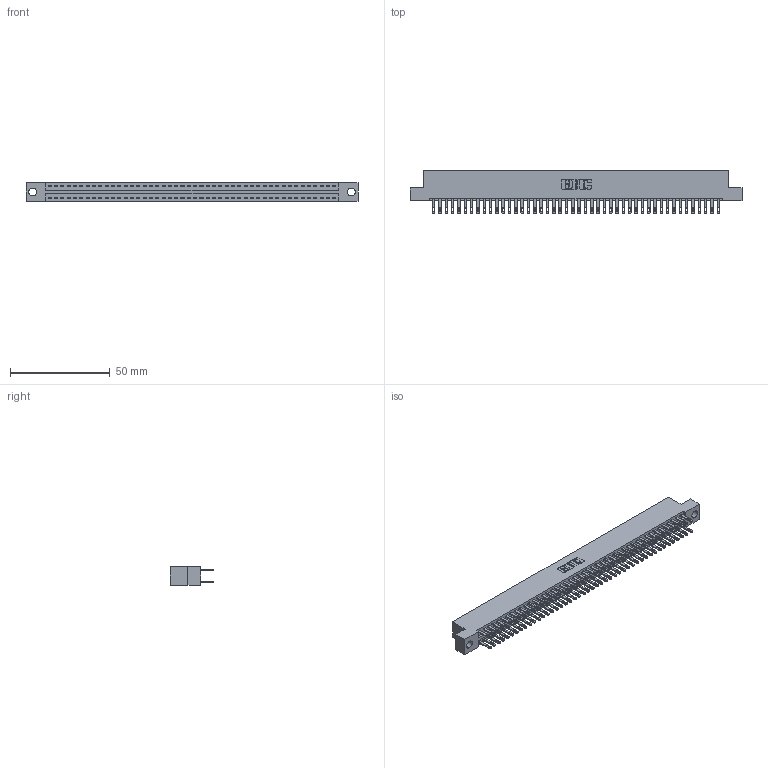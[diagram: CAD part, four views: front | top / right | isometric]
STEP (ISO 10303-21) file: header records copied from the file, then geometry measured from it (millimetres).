
FILE_DESCRIPTION (( 'STEP AP203' ), '1' );
FILE_NAME ('346-092-500-204.STEP', '2018-08-30T02:48:22', ( '' ), ( '' ), 'SwSTEP 2.0', 'SolidWorks 2016', '' );
FILE_SCHEMA (( 'CONFIG_CONTROL_DESIGN' ));
Length unit declared in the file: inch
Products named in the file (3): 346 Part_Flush Mounting Lugs - 0.156 Dia-TH; 345-292-001_345-293-100; 346-092-500-204
Assembly tree (93 placements, depth 2):
  346-092-500-204
    346 Part_Flush Mounting Lugs - 0.156 Dia-TH
    345-292-001_345-293-100  x92
Bounding box: 166.62 x 21.84 x 9.4 mm (x, y, z)
Volume: 16472.3 mm3; surface area: 23481.4 mm2
Topology: 93 solids, 93 shells, 4538 faces, 13853 edges, 9234 vertices
Faces by surface type: plane 2744, cylinder 1794
Entity records: 29415 total; most frequent: CARTESIAN_POINT 4840, ORIENTED_EDGE 4774, DIRECTION 4319, EDGE_CURVE 2387, LINE 2067, VECTOR 2067, VERTEX_POINT 1590, AXIS2_PLACEMENT_3D 1126
